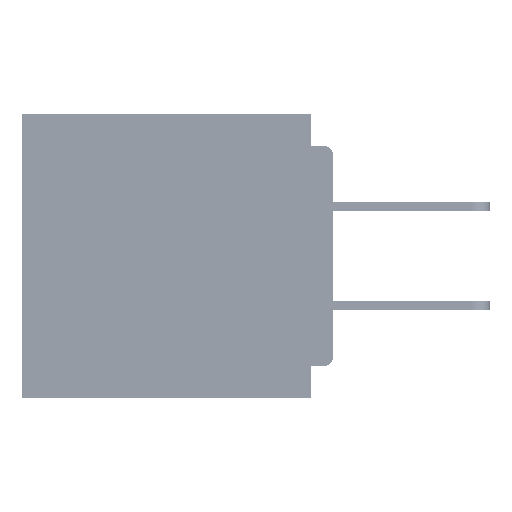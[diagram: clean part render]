
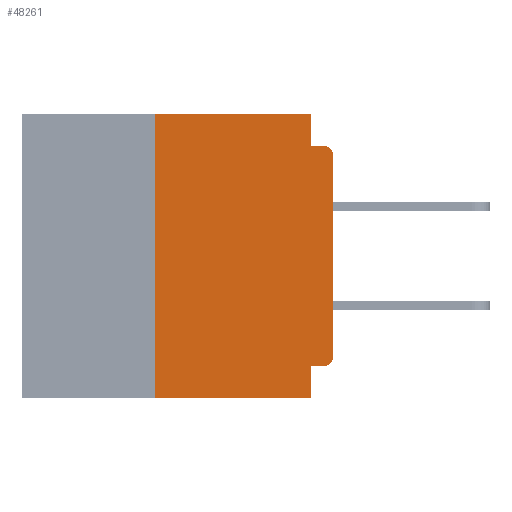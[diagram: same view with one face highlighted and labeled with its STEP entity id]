
A CAD part, left-side view. The second image highlights one B-rep face of the part: STEP entity #48261.
In plain terms, the highlighted planar face has unit normal (-1, 0, 0).
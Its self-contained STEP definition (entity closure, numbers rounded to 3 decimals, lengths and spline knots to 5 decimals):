
#178 = VERTEX_POINT ( 'NONE', #37717 ) ;
#268 = LINE ( 'NONE', #14337, #55540 ) ;
#570 = CARTESIAN_POINT ( 'NONE',  ( 0., 0.437, -0.4 ) ) ;
#1226 = LINE ( 'NONE', #38272, #29726 ) ;
#1992 = CARTESIAN_POINT ( 'NONE',  ( 0., 0., 0. ) ) ;
#2069 = ORIENTED_EDGE ( 'NONE', *, *, #19678, .T. ) ;
#3506 = AXIS2_PLACEMENT_3D ( 'NONE', #28823, #66130, #34209 ) ;
#4220 = ORIENTED_EDGE ( 'NONE', *, *, #37451, .F. ) ;
#6830 = LINE ( 'NONE', #19246, #46216 ) ;
#7415 = ORIENTED_EDGE ( 'NONE', *, *, #65947, .F. ) ;
#8445 = VECTOR ( 'NONE', #39334, 39.37008 ) ;
#8677 = LINE ( 'NONE', #570, #63863 ) ;
#11504 = CARTESIAN_POINT ( 'NONE',  ( 0., 0.25, -0.4 ) ) ;
#11554 = DIRECTION ( 'NONE',  ( 0., -1., 0. ) ) ;
#12551 = DIRECTION ( 'NONE',  ( -1., 0., 0. ) ) ;
#13888 = VECTOR ( 'NONE', #54121, 39.37008 ) ;
#14044 = EDGE_CURVE ( 'NONE', #57196, #23250, #64933, .T. ) ;
#14337 = CARTESIAN_POINT ( 'NONE',  ( 0., 0.031, 0. ) ) ;
#14440 = ORIENTED_EDGE ( 'NONE', *, *, #50458, .T. ) ;
#15003 = CARTESIAN_POINT ( 'NONE',  ( 0., 0.015, -0.045 ) ) ;
#15993 = CARTESIAN_POINT ( 'NONE',  ( 0., 0.031, -0.4 ) ) ;
#16055 = VERTEX_POINT ( 'NONE', #55346 ) ;
#18546 = CARTESIAN_POINT ( 'NONE',  ( 0., 0.031, -0.355 ) ) ;
#18951 = CARTESIAN_POINT ( 'NONE',  ( 0., 0., -0.06 ) ) ;
#19246 = CARTESIAN_POINT ( 'NONE',  ( 0., 0.25, -0.4 ) ) ;
#19343 = LINE ( 'NONE', #50350, #8445 ) ;
#19678 = EDGE_CURVE ( 'NONE', #27108, #178, #8677, .T. ) ;
#19873 = VERTEX_POINT ( 'NONE', #18546 ) ;
#20504 = DIRECTION ( 'NONE',  ( 0., 0., -1. ) ) ;
#21456 = EDGE_LOOP ( 'NONE', ( #14440, #38894, #7415, #37196, #40069, #4220, #2069, #32667, #49126, #66931 ) ) ;
#22025 = CARTESIAN_POINT ( 'NONE',  ( 0., 0., -0.355 ) ) ;
#22157 = CIRCLE ( 'NONE', #27259, 0.015 ) ;
#23250 = VERTEX_POINT ( 'NONE', #58558 ) ;
#26052 = AXIS2_PLACEMENT_3D ( 'NONE', #41846, #52590, #20504 ) ;
#26092 = VECTOR ( 'NONE', #58820, 39.37008 ) ;
#27108 = VERTEX_POINT ( 'NONE', #11504 ) ;
#27259 = AXIS2_PLACEMENT_3D ( 'NONE', #44663, #12551, #50059 ) ;
#28799 = CARTESIAN_POINT ( 'NONE',  ( 0., 0.031, -0.045 ) ) ;
#28823 = CARTESIAN_POINT ( 'NONE',  ( 0., 0.015, -0.34 ) ) ;
#29726 = VECTOR ( 'NONE', #11554, 39.37008 ) ;
#30023 = DIRECTION ( 'NONE',  ( 0., 0., 1. ) ) ;
#31893 = EDGE_CURVE ( 'NONE', #57196, #19873, #67339, .T. ) ;
#32667 = ORIENTED_EDGE ( 'NONE', *, *, #67699, .F. ) ;
#32692 = EDGE_CURVE ( 'NONE', #66793, #34233, #22157, .T. ) ;
#34209 = DIRECTION ( 'NONE',  ( 0., 0., -1. ) ) ;
#34233 = VERTEX_POINT ( 'NONE', #15003 ) ;
#34604 = EDGE_CURVE ( 'NONE', #16055, #48181, #19343, .T. ) ;
#35965 = CARTESIAN_POINT ( 'NONE',  ( 0., 0.015, -0.355 ) ) ;
#36961 = VECTOR ( 'NONE', #50233, 39.37008 ) ;
#37196 = ORIENTED_EDGE ( 'NONE', *, *, #42183, .F. ) ;
#37451 = EDGE_CURVE ( 'NONE', #27108, #16055, #6830, .T. ) ;
#37717 = CARTESIAN_POINT ( 'NONE',  ( 0., 0.031, -0.4 ) ) ;
#38272 = CARTESIAN_POINT ( 'NONE',  ( 0., 0., -0.045 ) ) ;
#38894 = ORIENTED_EDGE ( 'NONE', *, *, #32692, .T. ) ;
#39334 = DIRECTION ( 'NONE',  ( 0., -1., 0. ) ) ;
#40069 = ORIENTED_EDGE ( 'NONE', *, *, #34604, .F. ) ;
#41846 = CARTESIAN_POINT ( 'NONE',  ( 0., 0.437, 0. ) ) ;
#42183 = EDGE_CURVE ( 'NONE', #48181, #49294, #268, .T. ) ;
#44663 = CARTESIAN_POINT ( 'NONE',  ( 0., 0.015, -0.06 ) ) ;
#46216 = VECTOR ( 'NONE', #30023, 39.37008 ) ;
#46746 = CARTESIAN_POINT ( 'NONE',  ( 0., 0.031, 0. ) ) ;
#48181 = VERTEX_POINT ( 'NONE', #46746 ) ;
#48261 = ADVANCED_FACE ( 'NONE', ( #63350 ), #52359, .F. ) ;
#49126 = ORIENTED_EDGE ( 'NONE', *, *, #31893, .F. ) ;
#49294 = VERTEX_POINT ( 'NONE', #28799 ) ;
#50059 = DIRECTION ( 'NONE',  ( 0., 0., -1. ) ) ;
#50233 = DIRECTION ( 'NONE',  ( 0., 0., 1. ) ) ;
#50350 = CARTESIAN_POINT ( 'NONE',  ( 0., 0.437, 0. ) ) ;
#50458 = EDGE_CURVE ( 'NONE', #23250, #66793, #51213, .T. ) ;
#51213 = LINE ( 'NONE', #1992, #36961 ) ;
#52359 = PLANE ( 'NONE',  #26052 ) ;
#52590 = DIRECTION ( 'NONE',  ( 1., 0., 0. ) ) ;
#52927 = LINE ( 'NONE', #15993, #26092 ) ;
#54121 = DIRECTION ( 'NONE',  ( 0., 1., 0. ) ) ;
#55346 = CARTESIAN_POINT ( 'NONE',  ( 0., 0.25, 0. ) ) ;
#55540 = VECTOR ( 'NONE', #62490, 39.37008 ) ;
#57196 = VERTEX_POINT ( 'NONE', #35965 ) ;
#58558 = CARTESIAN_POINT ( 'NONE',  ( 0., 0., -0.34 ) ) ;
#58820 = DIRECTION ( 'NONE',  ( 0., 0., -1. ) ) ;
#59266 = DIRECTION ( 'NONE',  ( 0., -1., 0. ) ) ;
#62490 = DIRECTION ( 'NONE',  ( 0., 0., -1. ) ) ;
#63350 = FACE_OUTER_BOUND ( 'NONE', #21456, .T. ) ;
#63863 = VECTOR ( 'NONE', #59266, 39.37008 ) ;
#64933 = CIRCLE ( 'NONE', #3506, 0.015 ) ;
#65947 = EDGE_CURVE ( 'NONE', #49294, #34233, #1226, .T. ) ;
#66130 = DIRECTION ( 'NONE',  ( -1., 0., 0. ) ) ;
#66793 = VERTEX_POINT ( 'NONE', #18951 ) ;
#66931 = ORIENTED_EDGE ( 'NONE', *, *, #14044, .T. ) ;
#67339 = LINE ( 'NONE', #22025, #13888 ) ;
#67699 = EDGE_CURVE ( 'NONE', #19873, #178, #52927, .T. ) ;
